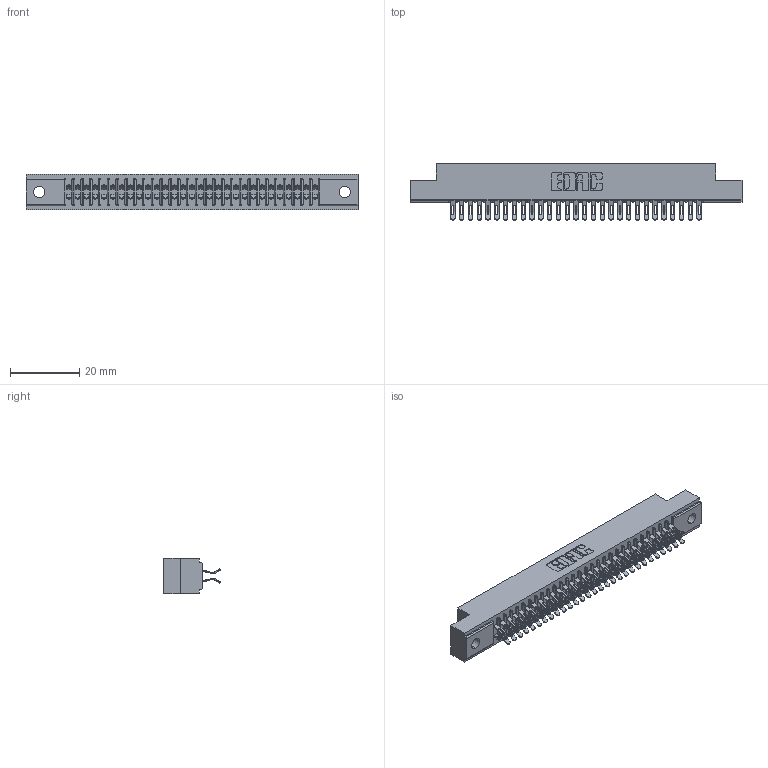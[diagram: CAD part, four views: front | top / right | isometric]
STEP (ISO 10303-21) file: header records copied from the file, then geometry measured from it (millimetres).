
FILE_DESCRIPTION (( 'STEP AP203' ), '1' );
FILE_NAME ('391-058-555-202.STEP', '2018-08-09T11:59:48', ( '' ), ( '' ), 'SwSTEP 2.0', 'SolidWorks 2016', '' );
FILE_SCHEMA (( 'CONFIG_CONTROL_DESIGN' ));
Length unit declared in the file: inch
Products named in the file (3): 341 Part_.128 (3.25) Dia Mounting Holes; 341-292-001_341-292-155; 391-058-555-202
Assembly tree (59 placements, depth 2):
  391-058-555-202
    341 Part_.128 (3.25) Dia Mounting Holes
    341-292-001_341-292-155  x58
Bounding box: 95.89 x 16.31 x 10.16 mm (x, y, z)
Volume: 7102.7 mm3; surface area: 12420.4 mm2
Topology: 59 solids, 59 shells, 4640 faces, 13859 edges, 9022 vertices
Faces by surface type: plane 2504, cylinder 2020, sphere 60, torus 56
Entity records: 37300 total; most frequent: CARTESIAN_POINT 6217, ORIENTED_EDGE 6166, DIRECTION 6033, EDGE_CURVE 3083, LINE 2461, VECTOR 2461, VERTEX_POINT 1954, AXIS2_PLACEMENT_3D 1786
